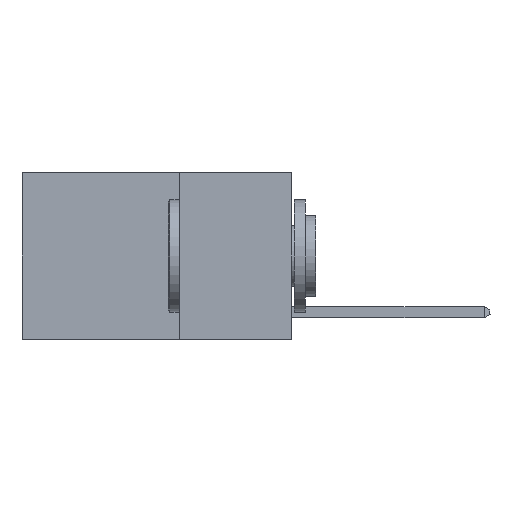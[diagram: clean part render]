
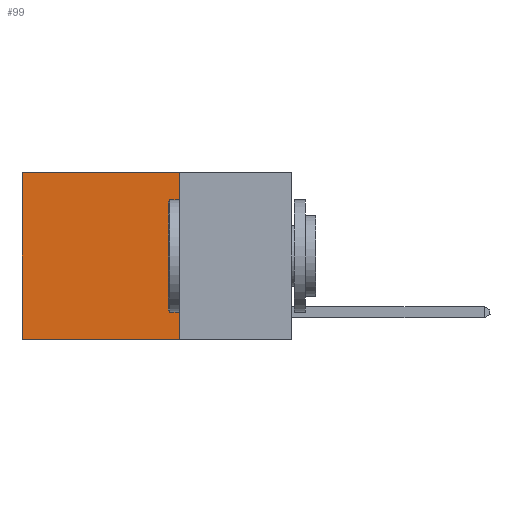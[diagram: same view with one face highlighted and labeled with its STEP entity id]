
A CAD part, left-side view. The second image highlights one B-rep face of the part: STEP entity #99.
In plain terms, the highlighted planar face has unit normal (-1, 0, 0).
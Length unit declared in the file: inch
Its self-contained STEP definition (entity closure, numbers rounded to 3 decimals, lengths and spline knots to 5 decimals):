
#33 = DIRECTION ( 'NONE',  ( 0., 1., 0. ) ) ;
#99 = ADVANCED_FACE ( 'NONE', ( #13470 ), #4059, .F. ) ;
#679 = VECTOR ( 'NONE', #17430, 39.37008 ) ;
#1199 = VECTOR ( 'NONE', #7891, 39.37008 ) ;
#1932 = VECTOR ( 'NONE', #33, 39.37008 ) ;
#2221 = ORIENTED_EDGE ( 'NONE', *, *, #5803, .F. ) ;
#2617 = AXIS2_PLACEMENT_3D ( 'NONE', #11871, #17338, #17007 ) ;
#3616 = CARTESIAN_POINT ( 'NONE',  ( 0.2625, 0.6, -0.37 ) ) ;
#4059 = PLANE ( 'NONE',  #2617 ) ;
#4081 = LINE ( 'NONE', #8258, #1932 ) ;
#4638 = VECTOR ( 'NONE', #5292, 39.37008 ) ;
#5020 = EDGE_CURVE ( 'NONE', #13988, #11489, #8508, .T. ) ;
#5056 = CARTESIAN_POINT ( 'NONE',  ( 0.2625, 0.25, 0. ) ) ;
#5292 = DIRECTION ( 'NONE',  ( 0., 0., -1. ) ) ;
#5351 = CARTESIAN_POINT ( 'NONE',  ( 0.2625, 0.25, 0. ) ) ;
#5803 = EDGE_CURVE ( 'NONE', #12781, #13972, #7451, .T. ) ;
#6044 = ORIENTED_EDGE ( 'NONE', *, *, #12952, .F. ) ;
#6585 = EDGE_LOOP ( 'NONE', ( #9599, #6044, #2221, #14471 ) ) ;
#7451 = LINE ( 'NONE', #5351, #4638 ) ;
#7605 = EDGE_CURVE ( 'NONE', #12781, #13988, #4081, .T. ) ;
#7891 = DIRECTION ( 'NONE',  ( 0., 0., -1. ) ) ;
#8258 = CARTESIAN_POINT ( 'NONE',  ( 0.2625, 0.25, 0. ) ) ;
#8508 = LINE ( 'NONE', #9213, #1199 ) ;
#9213 = CARTESIAN_POINT ( 'NONE',  ( 0.2625, 0.6, 0. ) ) ;
#9599 = ORIENTED_EDGE ( 'NONE', *, *, #5020, .T. ) ;
#11489 = VERTEX_POINT ( 'NONE', #3616 ) ;
#11505 = LINE ( 'NONE', #14731, #679 ) ;
#11871 = CARTESIAN_POINT ( 'NONE',  ( 0.2625, 0.25, 0. ) ) ;
#12781 = VERTEX_POINT ( 'NONE', #5056 ) ;
#12952 = EDGE_CURVE ( 'NONE', #13972, #11489, #11505, .T. ) ;
#13470 = FACE_OUTER_BOUND ( 'NONE', #6585, .T. ) ;
#13972 = VERTEX_POINT ( 'NONE', #15647 ) ;
#13988 = VERTEX_POINT ( 'NONE', #14359 ) ;
#14359 = CARTESIAN_POINT ( 'NONE',  ( 0.2625, 0.6, 0. ) ) ;
#14471 = ORIENTED_EDGE ( 'NONE', *, *, #7605, .T. ) ;
#14731 = CARTESIAN_POINT ( 'NONE',  ( 0.2625, 0.25, -0.37 ) ) ;
#15647 = CARTESIAN_POINT ( 'NONE',  ( 0.2625, 0.25, -0.37 ) ) ;
#17007 = DIRECTION ( 'NONE',  ( 0., 0., -1. ) ) ;
#17338 = DIRECTION ( 'NONE',  ( 1., 0., 0. ) ) ;
#17430 = DIRECTION ( 'NONE',  ( 0., 1., 0. ) ) ;
